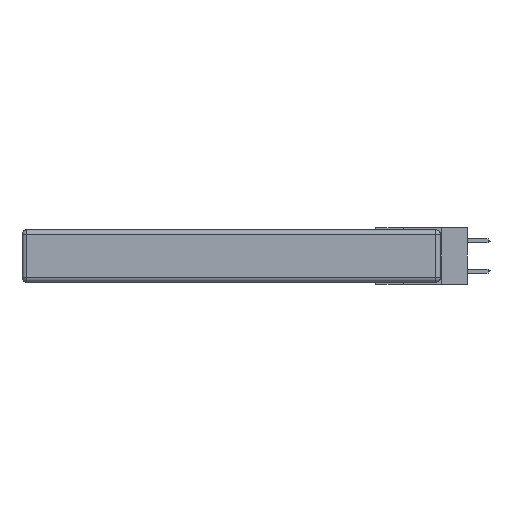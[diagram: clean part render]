
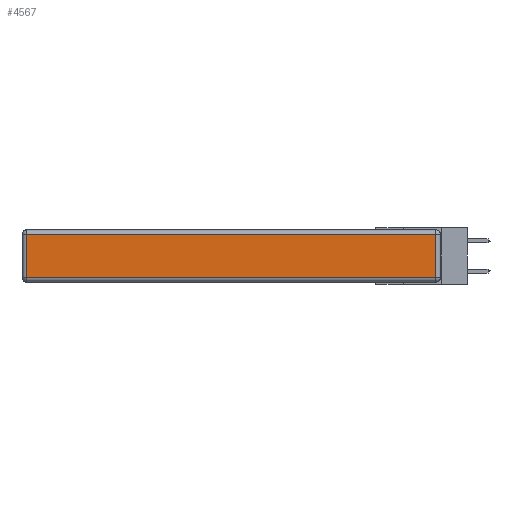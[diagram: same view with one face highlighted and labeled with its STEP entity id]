
A CAD part, left-side view. The second image highlights one B-rep face of the part: STEP entity #4567.
In plain terms, the highlighted planar face has unit normal (-1, 0, 0).
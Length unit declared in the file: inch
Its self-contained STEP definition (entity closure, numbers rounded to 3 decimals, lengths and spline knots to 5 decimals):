
#98 = DIRECTION ( 'NONE',  ( 0., 0., 1. ) ) ;
#354 = DIRECTION ( 'NONE',  ( 0., 0., -1. ) ) ;
#708 = CARTESIAN_POINT ( 'NONE',  ( 0., 2.72, -0.313 ) ) ;
#2465 = VECTOR ( 'NONE', #354, 39.37008 ) ;
#3017 = EDGE_CURVE ( 'NONE', #8146, #3087, #14301, .T. ) ;
#3087 = VERTEX_POINT ( 'NONE', #708 ) ;
#3150 = DIRECTION ( 'NONE',  ( 0., 0., 1. ) ) ;
#3590 = LINE ( 'NONE', #10078, #13893 ) ;
#3608 = EDGE_LOOP ( 'NONE', ( #11903, #15243, #20725, #4887 ) ) ;
#3687 = FACE_OUTER_BOUND ( 'NONE', #3608, .T. ) ;
#4567 = ADVANCED_FACE ( 'NONE', ( #3687 ), #8030, .T. ) ;
#4887 = ORIENTED_EDGE ( 'NONE', *, *, #3017, .T. ) ;
#4944 = DIRECTION ( 'NONE',  ( 0., 1., 0. ) ) ;
#6105 = DIRECTION ( 'NONE',  ( 0., -1., 0. ) ) ;
#6192 = VECTOR ( 'NONE', #3150, 39.37008 ) ;
#8030 = PLANE ( 'NONE',  #13810 ) ;
#8146 = VERTEX_POINT ( 'NONE', #15774 ) ;
#8771 = LINE ( 'NONE', #19533, #6192 ) ;
#9356 = CARTESIAN_POINT ( 'NONE',  ( 0., 0., -0.313 ) ) ;
#9646 = EDGE_CURVE ( 'NONE', #3087, #14239, #10087, .T. ) ;
#9896 = EDGE_CURVE ( 'NONE', #15963, #8146, #3590, .T. ) ;
#10078 = CARTESIAN_POINT ( 'NONE',  ( 0., 2.75, -0.03 ) ) ;
#10087 = LINE ( 'NONE', #9356, #13647 ) ;
#11903 = ORIENTED_EDGE ( 'NONE', *, *, #9646, .T. ) ;
#12706 = CARTESIAN_POINT ( 'NONE',  ( 0., 0.03, -0.313 ) ) ;
#13054 = DIRECTION ( 'NONE',  ( -1., 0., 0. ) ) ;
#13647 = VECTOR ( 'NONE', #6105, 39.37008 ) ;
#13746 = EDGE_CURVE ( 'NONE', #14239, #15963, #8771, .T. ) ;
#13778 = CARTESIAN_POINT ( 'NONE',  ( 0., 0.03, -0.03 ) ) ;
#13810 = AXIS2_PLACEMENT_3D ( 'NONE', #14619, #13054, #98 ) ;
#13893 = VECTOR ( 'NONE', #4944, 39.37008 ) ;
#14239 = VERTEX_POINT ( 'NONE', #12706 ) ;
#14301 = LINE ( 'NONE', #18186, #2465 ) ;
#14619 = CARTESIAN_POINT ( 'NONE',  ( 0., 0., -0.343 ) ) ;
#15243 = ORIENTED_EDGE ( 'NONE', *, *, #13746, .T. ) ;
#15774 = CARTESIAN_POINT ( 'NONE',  ( 0., 2.72, -0.03 ) ) ;
#15963 = VERTEX_POINT ( 'NONE', #13778 ) ;
#18186 = CARTESIAN_POINT ( 'NONE',  ( 0., 2.72, -0.343 ) ) ;
#19533 = CARTESIAN_POINT ( 'NONE',  ( 0., 0.03, -0.343 ) ) ;
#20725 = ORIENTED_EDGE ( 'NONE', *, *, #9896, .T. ) ;
